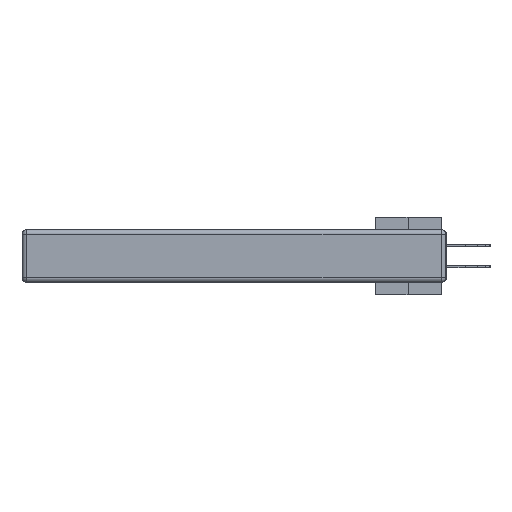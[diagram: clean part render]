
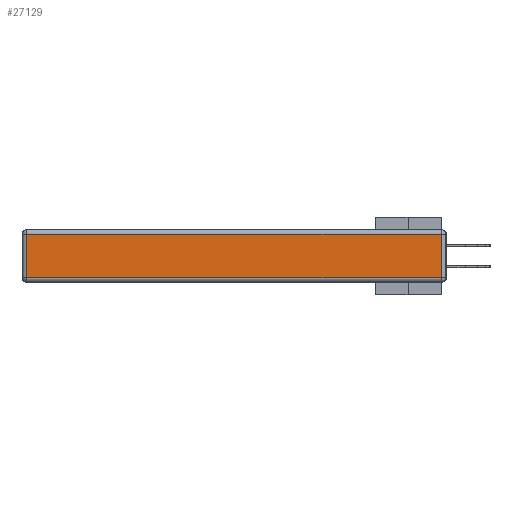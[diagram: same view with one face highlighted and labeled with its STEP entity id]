
A CAD part, left-side view. The second image highlights one B-rep face of the part: STEP entity #27129.
In plain terms, the highlighted planar face has unit normal (-1, 0, 0).
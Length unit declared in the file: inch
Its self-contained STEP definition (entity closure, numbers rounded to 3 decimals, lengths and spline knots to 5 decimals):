
#535 = VERTEX_POINT ( 'NONE', #14370 ) ;
#1673 = DIRECTION ( 'NONE',  ( 0., 1., 0. ) ) ;
#1737 = EDGE_CURVE ( 'NONE', #40347, #535, #20332, .T. ) ;
#4996 = VERTEX_POINT ( 'NONE', #19080 ) ;
#6449 = EDGE_LOOP ( 'NONE', ( #12297, #25264, #17474, #37714 ) ) ;
#9484 = CARTESIAN_POINT ( 'NONE',  ( 0., 2.72, -0.343 ) ) ;
#10605 = CARTESIAN_POINT ( 'NONE',  ( 0., 0.03, -0.343 ) ) ;
#10858 = LINE ( 'NONE', #10605, #19241 ) ;
#12297 = ORIENTED_EDGE ( 'NONE', *, *, #42328, .T. ) ;
#14370 = CARTESIAN_POINT ( 'NONE',  ( 0., 2.72, -0.03 ) ) ;
#15251 = CARTESIAN_POINT ( 'NONE',  ( 0., 0.03, -0.313 ) ) ;
#17056 = DIRECTION ( 'NONE',  ( -1., 0., 0. ) ) ;
#17474 = ORIENTED_EDGE ( 'NONE', *, *, #1737, .T. ) ;
#17678 = PLANE ( 'NONE',  #35319 ) ;
#19080 = CARTESIAN_POINT ( 'NONE',  ( 0., 2.72, -0.313 ) ) ;
#19241 = VECTOR ( 'NONE', #35607, 39.37008 ) ;
#19782 = DIRECTION ( 'NONE',  ( 0., 0., -1. ) ) ;
#20332 = LINE ( 'NONE', #22945, #43256 ) ;
#22844 = LINE ( 'NONE', #23972, #39551 ) ;
#22945 = CARTESIAN_POINT ( 'NONE',  ( 0., 2.75, -0.03 ) ) ;
#23972 = CARTESIAN_POINT ( 'NONE',  ( 0., 0., -0.313 ) ) ;
#24278 = DIRECTION ( 'NONE',  ( 0., 0., 1. ) ) ;
#25061 = FACE_OUTER_BOUND ( 'NONE', #6449, .T. ) ;
#25264 = ORIENTED_EDGE ( 'NONE', *, *, #44279, .T. ) ;
#27129 = ADVANCED_FACE ( 'NONE', ( #25061 ), #17678, .T. ) ;
#28036 = DIRECTION ( 'NONE',  ( 0., -1., 0. ) ) ;
#35319 = AXIS2_PLACEMENT_3D ( 'NONE', #42383, #17056, #24278 ) ;
#35607 = DIRECTION ( 'NONE',  ( 0., 0., 1. ) ) ;
#35838 = VECTOR ( 'NONE', #19782, 39.37008 ) ;
#37714 = ORIENTED_EDGE ( 'NONE', *, *, #41123, .T. ) ;
#39551 = VECTOR ( 'NONE', #28036, 39.37008 ) ;
#40347 = VERTEX_POINT ( 'NONE', #40691 ) ;
#40691 = CARTESIAN_POINT ( 'NONE',  ( 0., 0.03, -0.03 ) ) ;
#40854 = LINE ( 'NONE', #9484, #35838 ) ;
#41123 = EDGE_CURVE ( 'NONE', #535, #4996, #40854, .T. ) ;
#42328 = EDGE_CURVE ( 'NONE', #4996, #46297, #22844, .T. ) ;
#42383 = CARTESIAN_POINT ( 'NONE',  ( 0., 0., -0.343 ) ) ;
#43256 = VECTOR ( 'NONE', #1673, 39.37008 ) ;
#44279 = EDGE_CURVE ( 'NONE', #46297, #40347, #10858, .T. ) ;
#46297 = VERTEX_POINT ( 'NONE', #15251 ) ;
